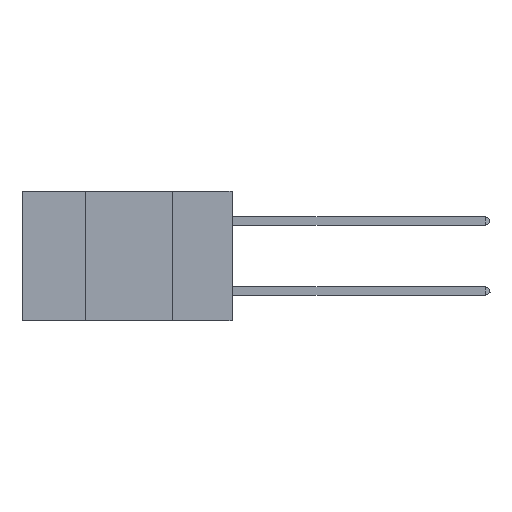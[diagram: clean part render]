
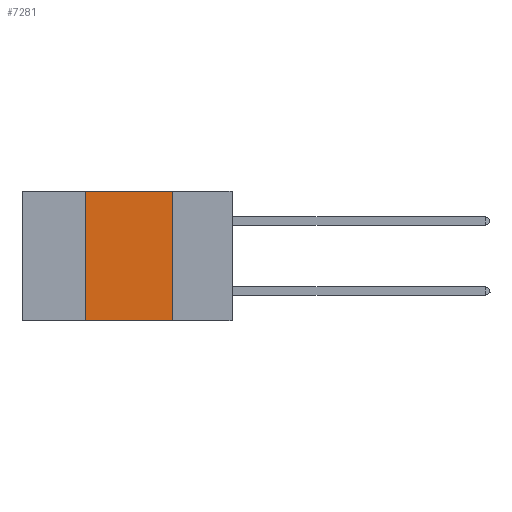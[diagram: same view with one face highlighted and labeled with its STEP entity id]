
A CAD part, left-side view. The second image highlights one B-rep face of the part: STEP entity #7281.
In plain terms, the highlighted planar face has unit normal (-1, 0, 0).
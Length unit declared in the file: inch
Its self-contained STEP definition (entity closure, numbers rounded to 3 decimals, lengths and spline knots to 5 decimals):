
#47 = VERTEX_POINT ( 'NONE', #20244 ) ;
#603 = DIRECTION ( 'NONE',  ( 0., 0., -1. ) ) ;
#1449 = LINE ( 'NONE', #17483, #11271 ) ;
#1552 = VECTOR ( 'NONE', #8260, 39.37008 ) ;
#2411 = CARTESIAN_POINT ( 'NONE',  ( 0., 0.6, 0. ) ) ;
#2465 = LINE ( 'NONE', #2411, #24758 ) ;
#2604 = PLANE ( 'NONE',  #23778 ) ;
#3394 = EDGE_CURVE ( 'NONE', #15552, #12447, #2465, .T. ) ;
#3734 = VERTEX_POINT ( 'NONE', #6009 ) ;
#4358 = DIRECTION ( 'NONE',  ( 0., -1., 0. ) ) ;
#4653 = CARTESIAN_POINT ( 'NONE',  ( 0., 0.42, 0. ) ) ;
#5396 = EDGE_LOOP ( 'NONE', ( #20390, #24512, #15047, #12008 ) ) ;
#5573 = CARTESIAN_POINT ( 'NONE',  ( 0., 0.17, 0. ) ) ;
#5965 = LINE ( 'NONE', #14548, #6578 ) ;
#6009 = CARTESIAN_POINT ( 'NONE',  ( 0., 0.17, -0.37 ) ) ;
#6578 = VECTOR ( 'NONE', #22352, 39.37008 ) ;
#7189 = EDGE_CURVE ( 'NONE', #47, #3734, #16239, .T. ) ;
#7281 = ADVANCED_FACE ( 'NONE', ( #16846 ), #2604, .F. ) ;
#8260 = DIRECTION ( 'NONE',  ( 0., -1., 0. ) ) ;
#8445 = CARTESIAN_POINT ( 'NONE',  ( 0., 0.6, 0. ) ) ;
#11271 = VECTOR ( 'NONE', #22989, 39.37008 ) ;
#12008 = ORIENTED_EDGE ( 'NONE', *, *, #7189, .T. ) ;
#12447 = VERTEX_POINT ( 'NONE', #5573 ) ;
#13097 = EDGE_CURVE ( 'NONE', #47, #15552, #1449, .T. ) ;
#14548 = CARTESIAN_POINT ( 'NONE',  ( 0., 0.17, 0. ) ) ;
#15047 = ORIENTED_EDGE ( 'NONE', *, *, #13097, .F. ) ;
#15552 = VERTEX_POINT ( 'NONE', #4653 ) ;
#16239 = LINE ( 'NONE', #19988, #1552 ) ;
#16846 = FACE_OUTER_BOUND ( 'NONE', #5396, .T. ) ;
#17483 = CARTESIAN_POINT ( 'NONE',  ( 0., 0.42, 0. ) ) ;
#19988 = CARTESIAN_POINT ( 'NONE',  ( 0., 0.6, -0.37 ) ) ;
#20244 = CARTESIAN_POINT ( 'NONE',  ( 0., 0.42, -0.37 ) ) ;
#20390 = ORIENTED_EDGE ( 'NONE', *, *, #21472, .F. ) ;
#21472 = EDGE_CURVE ( 'NONE', #12447, #3734, #5965, .T. ) ;
#22352 = DIRECTION ( 'NONE',  ( 0., 0., -1. ) ) ;
#22989 = DIRECTION ( 'NONE',  ( 0., 0., 1. ) ) ;
#23778 = AXIS2_PLACEMENT_3D ( 'NONE', #8445, #23946, #603 ) ;
#23946 = DIRECTION ( 'NONE',  ( 1., 0., 0. ) ) ;
#24512 = ORIENTED_EDGE ( 'NONE', *, *, #3394, .F. ) ;
#24758 = VECTOR ( 'NONE', #4358, 39.37008 ) ;
